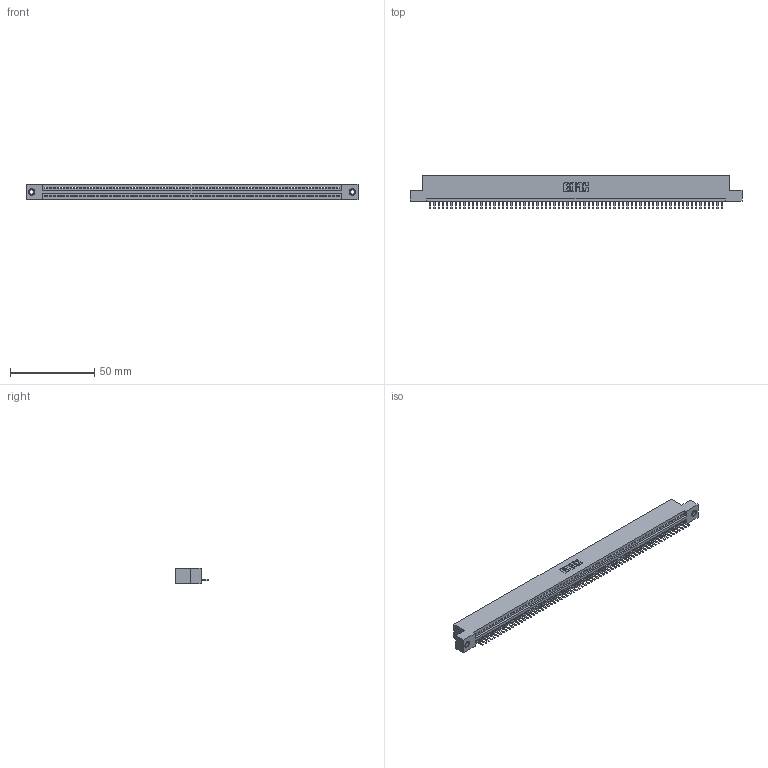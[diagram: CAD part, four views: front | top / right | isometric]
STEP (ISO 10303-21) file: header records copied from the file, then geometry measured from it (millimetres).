
FILE_DESCRIPTION (( 'STEP AP203' ), '1' );
FILE_NAME ('395-069-520-107.STEP', '2018-11-25T21:23:22', ( '' ), ( '' ), 'SwSTEP 2.0', 'SolidWorks 2016', '' );
FILE_SCHEMA (( 'CONFIG_CONTROL_DESIGN' ));
Length unit declared in the file: inch
Products named in the file (4): 345-292-001_345-293-120; 345-250-001_345-250-005-103; 345 Part_Flush Mounting Lugs - 0.156 Dia-TI; 395-069-520-107
Assembly tree (72 placements, depth 2):
  395-069-520-107
    345 Part_Flush Mounting Lugs - 0.156 Dia-TI
    345-292-001_345-293-120  x69
    345-250-001_345-250-005-103  x2
Bounding box: 196.47 x 19.68 x 9.4 mm (x, y, z)
Volume: 18670 mm3; surface area: 24560.9 mm2
Topology: 72 solids, 72 shells, 4464 faces, 13173 edges, 8590 vertices
Faces by surface type: plane 3010, cylinder 1438, cone 12, torus 4
Entity records: 49596 total; most frequent: CARTESIAN_POINT 8582, ORIENTED_EDGE 8566, DIRECTION 7471, EDGE_CURVE 4283, LINE 3851, VECTOR 3851, VERTEX_POINT 2848, AXIS2_PLACEMENT_3D 1810
